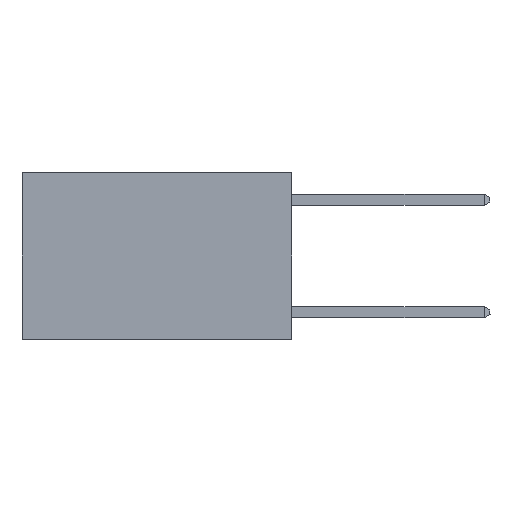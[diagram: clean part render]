
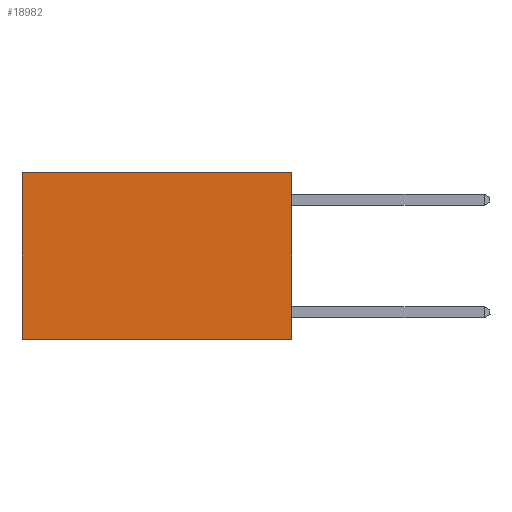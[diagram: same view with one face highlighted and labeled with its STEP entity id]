
A CAD part, left-side view. The second image highlights one B-rep face of the part: STEP entity #18982.
In plain terms, the highlighted planar face has unit normal (-1, 0, 0).
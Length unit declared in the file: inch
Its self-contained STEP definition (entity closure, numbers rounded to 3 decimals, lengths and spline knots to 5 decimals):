
#732 = AXIS2_PLACEMENT_3D ( 'NONE', #18964, #20591, #10589 ) ;
#1212 = VECTOR ( 'NONE', #2518, 39.37008 ) ;
#1235 = LINE ( 'NONE', #7714, #1212 ) ;
#1410 = CARTESIAN_POINT ( 'NONE',  ( 0.2625, 0., -0.37 ) ) ;
#1762 = DIRECTION ( 'NONE',  ( 0., 0., -1. ) ) ;
#2111 = LINE ( 'NONE', #11833, #18679 ) ;
#2518 = DIRECTION ( 'NONE',  ( 0., 1., 0. ) ) ;
#2866 = VERTEX_POINT ( 'NONE', #4789 ) ;
#3073 = LINE ( 'NONE', #1410, #7197 ) ;
#3710 = EDGE_CURVE ( 'NONE', #2866, #7525, #16430, .T. ) ;
#4643 = FACE_OUTER_BOUND ( 'NONE', #15236, .T. ) ;
#4789 = CARTESIAN_POINT ( 'NONE',  ( 0.2625, 0., 0. ) ) ;
#4901 = CARTESIAN_POINT ( 'NONE',  ( 0.2625, 0.6, -0.37 ) ) ;
#5820 = VERTEX_POINT ( 'NONE', #4901 ) ;
#6984 = EDGE_CURVE ( 'NONE', #2866, #20354, #1235, .T. ) ;
#7111 = PLANE ( 'NONE',  #732 ) ;
#7197 = VECTOR ( 'NONE', #10009, 39.37008 ) ;
#7525 = VERTEX_POINT ( 'NONE', #7690 ) ;
#7690 = CARTESIAN_POINT ( 'NONE',  ( 0.2625, 0., -0.37 ) ) ;
#7714 = CARTESIAN_POINT ( 'NONE',  ( 0.2625, 0., 0. ) ) ;
#8145 = EDGE_CURVE ( 'NONE', #7525, #5820, #3073, .T. ) ;
#10009 = DIRECTION ( 'NONE',  ( 0., 1., 0. ) ) ;
#10589 = DIRECTION ( 'NONE',  ( 0., 0., -1. ) ) ;
#11833 = CARTESIAN_POINT ( 'NONE',  ( 0.2625, 0.6, 0. ) ) ;
#13541 = DIRECTION ( 'NONE',  ( 0., 0., -1. ) ) ;
#13673 = CARTESIAN_POINT ( 'NONE',  ( 0.2625, 0., 0. ) ) ;
#14074 = CARTESIAN_POINT ( 'NONE',  ( 0.2625, 0.6, 0. ) ) ;
#15236 = EDGE_LOOP ( 'NONE', ( #18989, #19237, #19280, #19511 ) ) ;
#15691 = VECTOR ( 'NONE', #1762, 39.37008 ) ;
#16430 = LINE ( 'NONE', #13673, #15691 ) ;
#18679 = VECTOR ( 'NONE', #13541, 39.37008 ) ;
#18964 = CARTESIAN_POINT ( 'NONE',  ( 0.2625, 0., 0. ) ) ;
#18982 = ADVANCED_FACE ( 'NONE', ( #4643 ), #7111, .F. ) ;
#18989 = ORIENTED_EDGE ( 'NONE', *, *, #20791, .T. ) ;
#19237 = ORIENTED_EDGE ( 'NONE', *, *, #8145, .F. ) ;
#19280 = ORIENTED_EDGE ( 'NONE', *, *, #3710, .F. ) ;
#19511 = ORIENTED_EDGE ( 'NONE', *, *, #6984, .T. ) ;
#20354 = VERTEX_POINT ( 'NONE', #14074 ) ;
#20591 = DIRECTION ( 'NONE',  ( 1., 0., 0. ) ) ;
#20791 = EDGE_CURVE ( 'NONE', #20354, #5820, #2111, .T. ) ;
